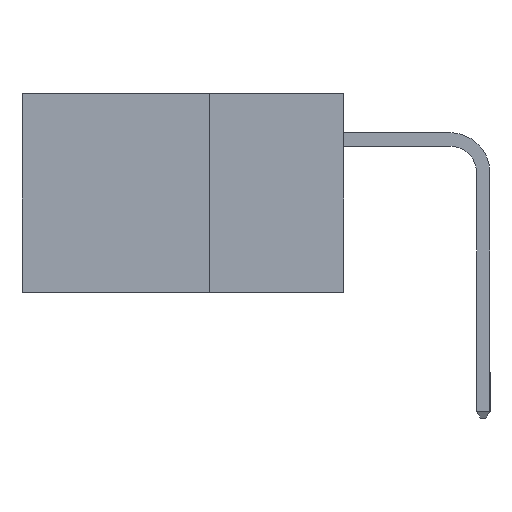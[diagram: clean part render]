
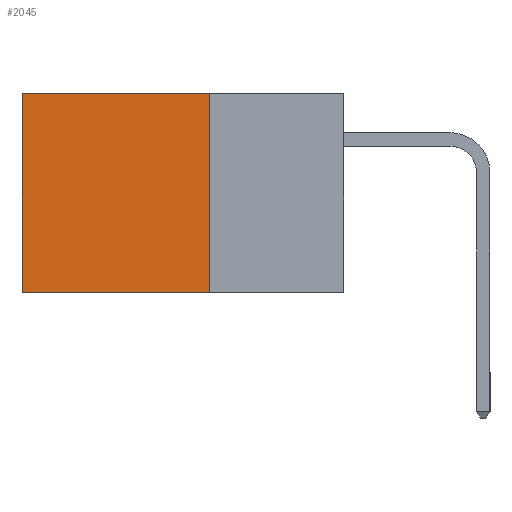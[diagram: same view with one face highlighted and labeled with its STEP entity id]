
A CAD part, left-side view. The second image highlights one B-rep face of the part: STEP entity #2045.
In plain terms, the highlighted planar face has unit normal (-1, 0, 0).
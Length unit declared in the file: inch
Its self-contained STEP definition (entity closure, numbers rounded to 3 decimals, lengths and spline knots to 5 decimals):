
#406 = CARTESIAN_POINT ( 'NONE',  ( 0.2615, 0.25, 0. ) ) ;
#642 = CARTESIAN_POINT ( 'NONE',  ( 0.2615, 0.25, -0.37 ) ) ;
#866 = FACE_OUTER_BOUND ( 'NONE', #13398, .T. ) ;
#1161 = ORIENTED_EDGE ( 'NONE', *, *, #2765, .T. ) ;
#1726 = CARTESIAN_POINT ( 'NONE',  ( 0.2615, 0.6, -0.37 ) ) ;
#2010 = VERTEX_POINT ( 'NONE', #5467 ) ;
#2045 = ADVANCED_FACE ( 'NONE', ( #866 ), #9725, .F. ) ;
#2415 = CARTESIAN_POINT ( 'NONE',  ( 0.2615, 0.25, -0.37 ) ) ;
#2765 = EDGE_CURVE ( 'NONE', #7373, #2010, #5202, .T. ) ;
#3196 = EDGE_CURVE ( 'NONE', #4784, #11376, #10793, .T. ) ;
#3963 = ORIENTED_EDGE ( 'NONE', *, *, #4603, .F. ) ;
#4603 = EDGE_CURVE ( 'NONE', #7373, #4784, #14260, .T. ) ;
#4629 = EDGE_CURVE ( 'NONE', #2010, #11376, #11941, .T. ) ;
#4784 = VERTEX_POINT ( 'NONE', #2415 ) ;
#5171 = VECTOR ( 'NONE', #5549, 39.37008 ) ;
#5202 = LINE ( 'NONE', #12849, #14653 ) ;
#5467 = CARTESIAN_POINT ( 'NONE',  ( 0.2615, 0.6, 0. ) ) ;
#5549 = DIRECTION ( 'NONE',  ( 0., 0., -1. ) ) ;
#6294 = CARTESIAN_POINT ( 'NONE',  ( 0.2615, 0.25, -0.37 ) ) ;
#6316 = CARTESIAN_POINT ( 'NONE',  ( 0.2615, 0.6, -0.37 ) ) ;
#7373 = VERTEX_POINT ( 'NONE', #406 ) ;
#8185 = DIRECTION ( 'NONE',  ( 0., 1., 0. ) ) ;
#8421 = DIRECTION ( 'NONE',  ( 0., 1., 0. ) ) ;
#8827 = ORIENTED_EDGE ( 'NONE', *, *, #4629, .T. ) ;
#9725 = PLANE ( 'NONE',  #10086 ) ;
#10086 = AXIS2_PLACEMENT_3D ( 'NONE', #6294, #11091, #13053 ) ;
#10793 = LINE ( 'NONE', #642, #12278 ) ;
#10817 = DIRECTION ( 'NONE',  ( 0., 0., -1. ) ) ;
#11091 = DIRECTION ( 'NONE',  ( 1., 0., 0. ) ) ;
#11376 = VERTEX_POINT ( 'NONE', #1726 ) ;
#11941 = LINE ( 'NONE', #6316, #12274 ) ;
#12274 = VECTOR ( 'NONE', #10817, 39.37008 ) ;
#12278 = VECTOR ( 'NONE', #8185, 39.37008 ) ;
#12849 = CARTESIAN_POINT ( 'NONE',  ( 0.2615, 0.25, 0. ) ) ;
#13053 = DIRECTION ( 'NONE',  ( 0., 0., -1. ) ) ;
#13398 = EDGE_LOOP ( 'NONE', ( #8827, #14382, #3963, #1161 ) ) ;
#13511 = CARTESIAN_POINT ( 'NONE',  ( 0.2615, 0.25, -0.37 ) ) ;
#14260 = LINE ( 'NONE', #13511, #5171 ) ;
#14382 = ORIENTED_EDGE ( 'NONE', *, *, #3196, .F. ) ;
#14653 = VECTOR ( 'NONE', #8421, 39.37008 ) ;
